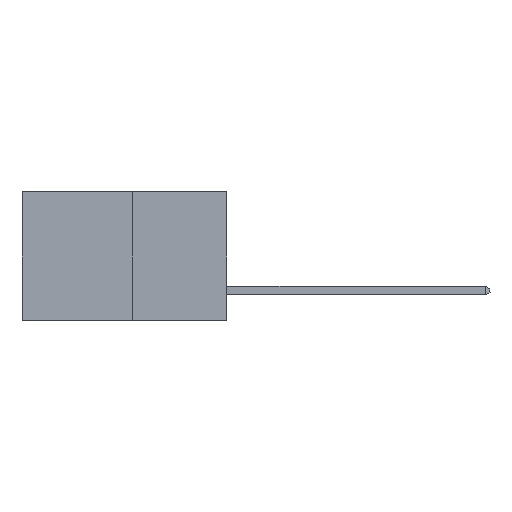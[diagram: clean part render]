
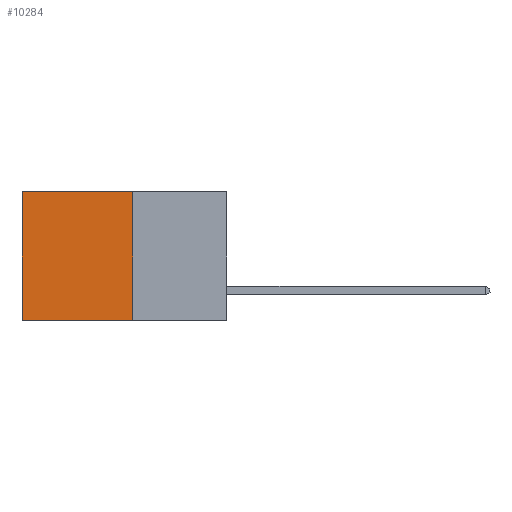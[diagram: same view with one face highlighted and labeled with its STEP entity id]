
A CAD part, left-side view. The second image highlights one B-rep face of the part: STEP entity #10284.
In plain terms, the highlighted planar face has unit normal (-1, 0, 0).
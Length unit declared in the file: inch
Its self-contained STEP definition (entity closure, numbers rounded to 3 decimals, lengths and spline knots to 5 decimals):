
#76 = EDGE_LOOP ( 'NONE', ( #1775, #1335, #1317, #1128 ) ) ;
#950 = DIRECTION ( 'NONE',  ( 0., 1., 0. ) ) ;
#1128 = ORIENTED_EDGE ( 'NONE', *, *, #10827, .T. ) ;
#1217 = FACE_OUTER_BOUND ( 'NONE', #76, .T. ) ;
#1317 = ORIENTED_EDGE ( 'NONE', *, *, #10441, .F. ) ;
#1335 = ORIENTED_EDGE ( 'NONE', *, *, #9574, .F. ) ;
#1775 = ORIENTED_EDGE ( 'NONE', *, *, #6549, .T. ) ;
#1801 = VERTEX_POINT ( 'NONE', #12102 ) ;
#2028 = VECTOR ( 'NONE', #950, 39.37008 ) ;
#2549 = LINE ( 'NONE', #2609, #8092 ) ;
#2609 = CARTESIAN_POINT ( 'NONE',  ( 0.277, 0.27, -0.37 ) ) ;
#3260 = CARTESIAN_POINT ( 'NONE',  ( 0.277, 0.27, -0.37 ) ) ;
#3350 = CARTESIAN_POINT ( 'NONE',  ( 0.277, 0.59, -0.37 ) ) ;
#3401 = DIRECTION ( 'NONE',  ( 0., 0., -1. ) ) ;
#3959 = VERTEX_POINT ( 'NONE', #6097 ) ;
#4223 = CARTESIAN_POINT ( 'NONE',  ( 0.277, 0.27, 0. ) ) ;
#6097 = CARTESIAN_POINT ( 'NONE',  ( 0.277, 0.59, -0.37 ) ) ;
#6549 = EDGE_CURVE ( 'NONE', #12729, #3959, #13774, .T. ) ;
#6553 = DIRECTION ( 'NONE',  ( 0., 1., 0. ) ) ;
#6812 = CARTESIAN_POINT ( 'NONE',  ( 0.277, 0.59, 0. ) ) ;
#7675 = DIRECTION ( 'NONE',  ( 0., 0., -1. ) ) ;
#8092 = VECTOR ( 'NONE', #9234, 39.37008 ) ;
#8199 = VERTEX_POINT ( 'NONE', #4223 ) ;
#8472 = VECTOR ( 'NONE', #6553, 39.37008 ) ;
#9234 = DIRECTION ( 'NONE',  ( 0., 0., -1. ) ) ;
#9574 = EDGE_CURVE ( 'NONE', #1801, #3959, #11068, .T. ) ;
#10284 = ADVANCED_FACE ( 'NONE', ( #1217 ), #13116, .F. ) ;
#10441 = EDGE_CURVE ( 'NONE', #8199, #1801, #2549, .T. ) ;
#10827 = EDGE_CURVE ( 'NONE', #8199, #12729, #13719, .T. ) ;
#11068 = LINE ( 'NONE', #13087, #8472 ) ;
#12102 = CARTESIAN_POINT ( 'NONE',  ( 0.277, 0.27, -0.37 ) ) ;
#12729 = VERTEX_POINT ( 'NONE', #6812 ) ;
#13087 = CARTESIAN_POINT ( 'NONE',  ( 0.277, 0.27, -0.37 ) ) ;
#13116 = PLANE ( 'NONE',  #14409 ) ;
#13719 = LINE ( 'NONE', #14208, #2028 ) ;
#13774 = LINE ( 'NONE', #3350, #14414 ) ;
#14156 = DIRECTION ( 'NONE',  ( 1., 0., 0. ) ) ;
#14208 = CARTESIAN_POINT ( 'NONE',  ( 0.277, 0.27, 0. ) ) ;
#14409 = AXIS2_PLACEMENT_3D ( 'NONE', #3260, #14156, #7675 ) ;
#14414 = VECTOR ( 'NONE', #3401, 39.37008 ) ;
